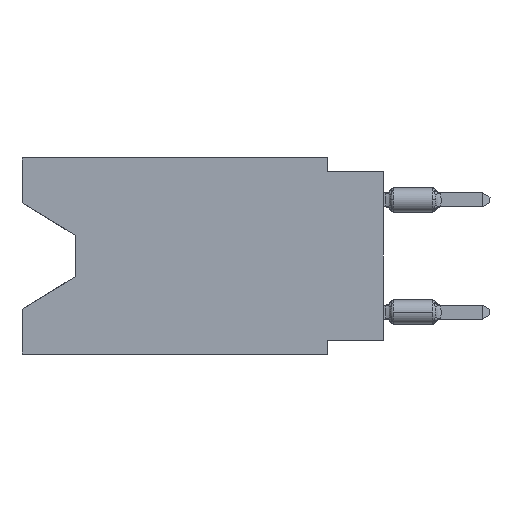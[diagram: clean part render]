
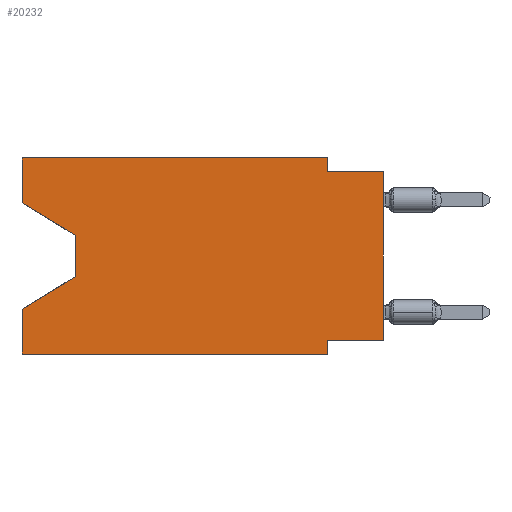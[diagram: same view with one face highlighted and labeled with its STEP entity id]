
A CAD part, left-side view. The second image highlights one B-rep face of the part: STEP entity #20232.
In plain terms, the highlighted planar face has unit normal (-1, 0, 0).
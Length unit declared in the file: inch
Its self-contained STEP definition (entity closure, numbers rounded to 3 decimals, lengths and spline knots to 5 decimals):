
#1 = VERTEX_POINT ( 'NONE', #1092 ) ;
#165 = DIRECTION ( 'NONE',  ( 0., 0., 1. ) ) ;
#176 = EDGE_CURVE ( 'NONE', #571, #15945, #20282, .T. ) ;
#233 = DIRECTION ( 'NONE',  ( 0., -1., 0. ) ) ;
#258 = VECTOR ( 'NONE', #4900, 39.37008 ) ;
#509 = VERTEX_POINT ( 'NONE', #6290 ) ;
#571 = VERTEX_POINT ( 'NONE', #3315 ) ;
#608 = ORIENTED_EDGE ( 'NONE', *, *, #7778, .T. ) ;
#736 = CARTESIAN_POINT ( 'NONE',  ( 0., 0.1, -0.35 ) ) ;
#919 = CARTESIAN_POINT ( 'NONE',  ( 0., 0.1, -0.325 ) ) ;
#1092 = CARTESIAN_POINT ( 'NONE',  ( 0., 0.1, 0. ) ) ;
#1186 = VERTEX_POINT ( 'NONE', #16528 ) ;
#1447 = LINE ( 'NONE', #6266, #12097 ) ;
#2161 = CARTESIAN_POINT ( 'NONE',  ( 0., 0.1, -0.025 ) ) ;
#3043 = ORIENTED_EDGE ( 'NONE', *, *, #176, .T. ) ;
#3225 = EDGE_CURVE ( 'NONE', #13930, #15657, #9558, .T. ) ;
#3267 = LINE ( 'NONE', #8084, #8381 ) ;
#3315 = CARTESIAN_POINT ( 'NONE',  ( 0., 0., -0.325 ) ) ;
#3610 = ORIENTED_EDGE ( 'NONE', *, *, #15216, .F. ) ;
#4212 = EDGE_CURVE ( 'NONE', #4576, #15657, #14130, .T. ) ;
#4329 = DIRECTION ( 'NONE',  ( 0., -1., 0. ) ) ;
#4341 = ORIENTED_EDGE ( 'NONE', *, *, #4212, .F. ) ;
#4355 = VECTOR ( 'NONE', #16714, 39.37008 ) ;
#4367 = LINE ( 'NONE', #12380, #14119 ) ;
#4377 = CARTESIAN_POINT ( 'NONE',  ( 0., 0.55, -0.138 ) ) ;
#4576 = VERTEX_POINT ( 'NONE', #17498 ) ;
#4900 = DIRECTION ( 'NONE',  ( 0., 0., -1. ) ) ;
#5049 = LINE ( 'NONE', #8442, #6050 ) ;
#5147 = VERTEX_POINT ( 'NONE', #2161 ) ;
#5862 = CARTESIAN_POINT ( 'NONE',  ( 0., 0.55, -0.212 ) ) ;
#6050 = VECTOR ( 'NONE', #233, 39.37008 ) ;
#6266 = CARTESIAN_POINT ( 'NONE',  ( 0., 0.1, 0. ) ) ;
#6290 = CARTESIAN_POINT ( 'NONE',  ( 0., 0.645, -0.08025 ) ) ;
#6475 = CARTESIAN_POINT ( 'NONE',  ( 0., 0.55, -0.212 ) ) ;
#6720 = CARTESIAN_POINT ( 'NONE',  ( 0., 0.645, 0. ) ) ;
#7187 = EDGE_CURVE ( 'NONE', #20086, #1, #12128, .T. ) ;
#7368 = PLANE ( 'NONE',  #17228 ) ;
#7393 = CARTESIAN_POINT ( 'NONE',  ( 0., 0.645, 0. ) ) ;
#7555 = CARTESIAN_POINT ( 'NONE',  ( 0., 0.645, -0.08025 ) ) ;
#7653 = DIRECTION ( 'NONE',  ( 0., 1., 0. ) ) ;
#7778 = EDGE_CURVE ( 'NONE', #1186, #13930, #15183, .T. ) ;
#7796 = CARTESIAN_POINT ( 'NONE',  ( 0., 0.645, -0.26975 ) ) ;
#7837 = ORIENTED_EDGE ( 'NONE', *, *, #19586, .T. ) ;
#8016 = VECTOR ( 'NONE', #13574, 39.37008 ) ;
#8084 = CARTESIAN_POINT ( 'NONE',  ( 0., 0., -0.025 ) ) ;
#8284 = CARTESIAN_POINT ( 'NONE',  ( 0., 0.1, -0.35 ) ) ;
#8381 = VECTOR ( 'NONE', #12711, 39.37008 ) ;
#8442 = CARTESIAN_POINT ( 'NONE',  ( 0., 0.645, -0.35 ) ) ;
#8758 = VERTEX_POINT ( 'NONE', #736 ) ;
#9558 = LINE ( 'NONE', #6475, #12272 ) ;
#9647 = DIRECTION ( 'NONE',  ( 0., 0., -1. ) ) ;
#10142 = EDGE_CURVE ( 'NONE', #509, #1186, #10623, .T. ) ;
#10623 = LINE ( 'NONE', #7555, #4355 ) ;
#11130 = DIRECTION ( 'NONE',  ( 1., 0., 0. ) ) ;
#11229 = FACE_OUTER_BOUND ( 'NONE', #18947, .T. ) ;
#11429 = ORIENTED_EDGE ( 'NONE', *, *, #19698, .F. ) ;
#11582 = CARTESIAN_POINT ( 'NONE',  ( 0., 0.645, 0. ) ) ;
#12097 = VECTOR ( 'NONE', #9647, 39.37008 ) ;
#12128 = LINE ( 'NONE', #12339, #18590 ) ;
#12152 = ORIENTED_EDGE ( 'NONE', *, *, #10142, .T. ) ;
#12272 = VECTOR ( 'NONE', #18998, 39.37008 ) ;
#12339 = CARTESIAN_POINT ( 'NONE',  ( 0., 0.645, 0. ) ) ;
#12380 = CARTESIAN_POINT ( 'NONE',  ( 0., 0., -0.325 ) ) ;
#12711 = DIRECTION ( 'NONE',  ( 0., -1., 0. ) ) ;
#13143 = ORIENTED_EDGE ( 'NONE', *, *, #3225, .T. ) ;
#13574 = DIRECTION ( 'NONE',  ( 0., 0., 1. ) ) ;
#13930 = VERTEX_POINT ( 'NONE', #5862 ) ;
#14043 = EDGE_CURVE ( 'NONE', #1, #5147, #1447, .T. ) ;
#14119 = VECTOR ( 'NONE', #7653, 39.37008 ) ;
#14130 = LINE ( 'NONE', #6720, #19708 ) ;
#14133 = VECTOR ( 'NONE', #14361, 39.37008 ) ;
#14336 = DIRECTION ( 'NONE',  ( 0., 0., 1. ) ) ;
#14361 = DIRECTION ( 'NONE',  ( 0., 0., -1. ) ) ;
#14833 = EDGE_CURVE ( 'NONE', #571, #20088, #4367, .T. ) ;
#15142 = ORIENTED_EDGE ( 'NONE', *, *, #7187, .F. ) ;
#15183 = LINE ( 'NONE', #4377, #258 ) ;
#15216 = EDGE_CURVE ( 'NONE', #20088, #8758, #18968, .T. ) ;
#15570 = CARTESIAN_POINT ( 'NONE',  ( 0., 0., 0. ) ) ;
#15657 = VERTEX_POINT ( 'NONE', #7796 ) ;
#15945 = VERTEX_POINT ( 'NONE', #19699 ) ;
#16212 = EDGE_CURVE ( 'NONE', #5147, #15945, #3267, .T. ) ;
#16451 = LINE ( 'NONE', #7393, #8016 ) ;
#16528 = CARTESIAN_POINT ( 'NONE',  ( 0., 0.55, -0.138 ) ) ;
#16714 = DIRECTION ( 'NONE',  ( 0., -0.855, -0.519 ) ) ;
#16822 = CARTESIAN_POINT ( 'NONE',  ( 0., 0.645, 0. ) ) ;
#17228 = AXIS2_PLACEMENT_3D ( 'NONE', #16822, #11130, #18732 ) ;
#17498 = CARTESIAN_POINT ( 'NONE',  ( 0., 0.645, -0.35 ) ) ;
#18441 = ORIENTED_EDGE ( 'NONE', *, *, #14043, .F. ) ;
#18583 = ORIENTED_EDGE ( 'NONE', *, *, #16212, .F. ) ;
#18590 = VECTOR ( 'NONE', #4329, 39.37008 ) ;
#18614 = ORIENTED_EDGE ( 'NONE', *, *, #14833, .F. ) ;
#18732 = DIRECTION ( 'NONE',  ( 0., 0., -1. ) ) ;
#18947 = EDGE_LOOP ( 'NONE', ( #12152, #608, #13143, #4341, #7837, #3610, #18614, #3043, #18583, #18441, #15142, #11429 ) ) ;
#18968 = LINE ( 'NONE', #8284, #14133 ) ;
#18990 = VECTOR ( 'NONE', #14336, 39.37008 ) ;
#18998 = DIRECTION ( 'NONE',  ( 0., 0.855, -0.519 ) ) ;
#19586 = EDGE_CURVE ( 'NONE', #4576, #8758, #5049, .T. ) ;
#19698 = EDGE_CURVE ( 'NONE', #509, #20086, #16451, .T. ) ;
#19699 = CARTESIAN_POINT ( 'NONE',  ( 0., 0., -0.025 ) ) ;
#19708 = VECTOR ( 'NONE', #165, 39.37008 ) ;
#20086 = VERTEX_POINT ( 'NONE', #11582 ) ;
#20088 = VERTEX_POINT ( 'NONE', #919 ) ;
#20232 = ADVANCED_FACE ( 'NONE', ( #11229 ), #7368, .F. ) ;
#20282 = LINE ( 'NONE', #15570, #18990 ) ;
